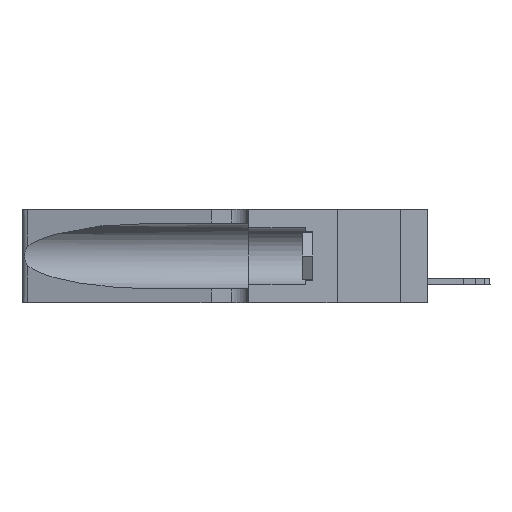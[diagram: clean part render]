
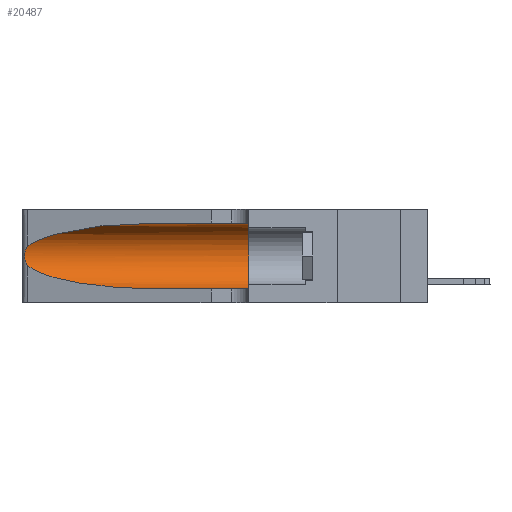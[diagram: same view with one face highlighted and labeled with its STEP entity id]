
A CAD part, left-side view. The second image highlights one B-rep face of the part: STEP entity #20487.
In plain terms, the highlighted cylindrical face has radius 3.308 mm (diameter 6.617 mm), a partial arc.
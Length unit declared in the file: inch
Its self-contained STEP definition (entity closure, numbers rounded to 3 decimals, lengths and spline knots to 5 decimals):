
#1 = CARTESIAN_POINT ( 'NONE',  ( 0.25555, 1.22994, 0.2215 ) ) ;
#87 = CARTESIAN_POINT ( 'NONE',  ( 0.1305, 0.35, 0.185 ) ) ;
#368 = B_SPLINE_CURVE_WITH_KNOTS ( 'NONE', 3,
 ( #2170, #1, #12106, #12592, #8756, #17978, #19268, #5569, #2104, #13566, #16265, #23050, #21181, #4207 ),
 .UNSPECIFIED., .F., .F.,
 ( 4, 2, 2, 2, 2, 2, 4 ),
 ( 0., 0.00027, 0.00053, 0.00107, 0.0016, 0.00187, 0.00214 ),
 .UNSPECIFIED. ) ;
#1150 = AXIS2_PLACEMENT_3D ( 'NONE', #9232, #19869, #3007 ) ;
#2104 = CARTESIAN_POINT ( 'NONE',  ( 0.26017, 1.23833, 0.17102 ) ) ;
#2170 = CARTESIAN_POINT ( 'NONE',  ( 0.25487, 1.22718, 0.22369 ) ) ;
#2233 = EDGE_CURVE ( 'NONE', #18518, #26636, #19519, .T. ) ;
#2275 = CARTESIAN_POINT ( 'NONE',  ( 0.18966, 0.96281, 0.31525 ) ) ;
#2387 = CARTESIAN_POINT ( 'NONE',  ( 0.18966, 0.96281, 0.05475 ) ) ;
#2442 = CARTESIAN_POINT ( 'NONE',  ( 0.25487, 1.22718, 0.14631 ) ) ;
#2450 = CARTESIAN_POINT ( 'NONE',  ( 0.25487, 1.22718, 0.22369 ) ) ;
#2698 = EDGE_CURVE ( 'NONE', #15589, #18518, #368, .T. ) ;
#3007 = DIRECTION ( 'NONE',  ( 0., 0., -1. ) ) ;
#3049 = CARTESIAN_POINT ( 'NONE',  ( 0.1305, 0.72297, 0.05475 ) ) ;
#4207 = CARTESIAN_POINT ( 'NONE',  ( 0.25487, 1.22718, 0.14631 ) ) ;
#4606 = ORIENTED_EDGE ( 'NONE', *, *, #25738, .F. ) ;
#5569 = CARTESIAN_POINT ( 'NONE',  ( 0.26075, 1.23896, 0.178 ) ) ;
#6267 = VERTEX_POINT ( 'NONE', #27074 ) ;
#6815 = VERTEX_POINT ( 'NONE', #14926 ) ;
#8517 = VECTOR ( 'NONE', #13620, 39.37008 ) ;
#8756 = CARTESIAN_POINT ( 'NONE',  ( 0.25854, 1.2359, 0.20912 ) ) ;
#9232 = CARTESIAN_POINT ( 'NONE',  ( 0.1305, 1.61858, 0.185 ) ) ;
#9313 = CARTESIAN_POINT ( 'NONE',  ( 0.1305, 1.61858, 0.05475 ) ) ;
#9803 = FACE_OUTER_BOUND ( 'NONE', #13865, .T. ) ;
#9966 = ORIENTED_EDGE ( 'NONE', *, *, #25538, .F. ) ;
#10868 = CARTESIAN_POINT ( 'NONE',  ( 0.25487, 1.22718, 0.14631 ) ) ;
#11461 = ORIENTED_EDGE ( 'NONE', *, *, #26034, .T. ) ;
#11840 = CIRCLE ( 'NONE', #14511, 0.13025 ) ;
#12106 = CARTESIAN_POINT ( 'NONE',  ( 0.25639, 1.23184, 0.21858 ) ) ;
#12592 = CARTESIAN_POINT ( 'NONE',  ( 0.25787, 1.23484, 0.2124 ) ) ;
#13566 = CARTESIAN_POINT ( 'NONE',  ( 0.25856, 1.23593, 0.16098 ) ) ;
#13620 = DIRECTION ( 'NONE',  ( 0., -1., 0. ) ) ;
#13839 = LINE ( 'NONE', #9313, #8517 ) ;
#13865 = EDGE_LOOP ( 'NONE', ( #27558, #18301, #23616, #11461, #4606, #9966 ) ) ;
#14511 = AXIS2_PLACEMENT_3D ( 'NONE', #87, #16988, #17082 ) ;
#14576 = LINE ( 'NONE', #24652, #18218 ) ;
#14824 = CYLINDRICAL_SURFACE ( 'NONE', #1150, 0.13025 ) ;
#14926 = CARTESIAN_POINT ( 'NONE',  ( 0.1305, 0.35, 0.31525 ) ) ;
#15065 = CARTESIAN_POINT ( 'NONE',  ( 0.1305, 0.72297, 0.31525 ) ) ;
#15589 = VERTEX_POINT ( 'NONE', #22653 ) ;
#16265 = CARTESIAN_POINT ( 'NONE',  ( 0.25789, 1.23486, 0.15765 ) ) ;
#16988 = DIRECTION ( 'NONE',  ( 0., 1., 0. ) ) ;
#17082 = DIRECTION ( 'NONE',  ( 0., 0., 1. ) ) ;
#17089 = CARTESIAN_POINT ( 'NONE',  ( 0.2373, 1.15595, 0.28018 ) ) ;
#17588 = CARTESIAN_POINT ( 'NONE',  ( 0.2373, 1.15595, 0.08982 ) ) ;
#17816 =( BOUNDED_CURVE ( )  B_SPLINE_CURVE ( 3, ( #15065, #2275, #17089, #2450 ),
 .UNSPECIFIED., .F., .F. ) 
 B_SPLINE_CURVE_WITH_KNOTS ( ( 4, 4 ),
 ( 1.5708, 2.84003 ),
 .UNSPECIFIED. ) 
 CURVE ( )  GEOMETRIC_REPRESENTATION_ITEM ( )  RATIONAL_B_SPLINE_CURVE ( ( 1., 0.87, 0.87, 1. ) ) 
 REPRESENTATION_ITEM ( '' )  );
#17978 = CARTESIAN_POINT ( 'NONE',  ( 0.26018, 1.23835, 0.19895 ) ) ;
#18218 = VECTOR ( 'NONE', #27413, 39.37008 ) ;
#18301 = ORIENTED_EDGE ( 'NONE', *, *, #2698, .T. ) ;
#18518 = VERTEX_POINT ( 'NONE', #2442 ) ;
#18757 = VERTEX_POINT ( 'NONE', #24623 ) ;
#19268 = CARTESIAN_POINT ( 'NONE',  ( 0.26075, 1.23896, 0.19203 ) ) ;
#19519 =( BOUNDED_CURVE ( )  B_SPLINE_CURVE ( 3, ( #10868, #17588, #2387, #21607 ),
 .UNSPECIFIED., .F., .T. ) 
 B_SPLINE_CURVE_WITH_KNOTS ( ( 4, 4 ),
 ( 3.44316, 4.71239 ),
 .UNSPECIFIED. ) 
 CURVE ( )  GEOMETRIC_REPRESENTATION_ITEM ( )  RATIONAL_B_SPLINE_CURVE ( ( 1., 0.87, 0.87, 1. ) ) 
 REPRESENTATION_ITEM ( '' )  );
#19869 = DIRECTION ( 'NONE',  ( 0., -1., 0. ) ) ;
#20487 = ADVANCED_FACE ( 'NONE', ( #9803 ), #14824, .F. ) ;
#21116 = EDGE_CURVE ( 'NONE', #18757, #15589, #17816, .T. ) ;
#21181 = CARTESIAN_POINT ( 'NONE',  ( 0.25555, 1.22993, 0.14849 ) ) ;
#21607 = CARTESIAN_POINT ( 'NONE',  ( 0.1305, 0.72297, 0.05475 ) ) ;
#22653 = CARTESIAN_POINT ( 'NONE',  ( 0.25487, 1.22718, 0.22369 ) ) ;
#23050 = CARTESIAN_POINT ( 'NONE',  ( 0.25639, 1.23186, 0.15144 ) ) ;
#23616 = ORIENTED_EDGE ( 'NONE', *, *, #2233, .T. ) ;
#24623 = CARTESIAN_POINT ( 'NONE',  ( 0.1305, 0.72297, 0.31525 ) ) ;
#24652 = CARTESIAN_POINT ( 'NONE',  ( 0.1305, 1.61858, 0.31525 ) ) ;
#25538 = EDGE_CURVE ( 'NONE', #18757, #6815, #14576, .T. ) ;
#25738 = EDGE_CURVE ( 'NONE', #6815, #6267, #11840, .T. ) ;
#26034 = EDGE_CURVE ( 'NONE', #26636, #6267, #13839, .T. ) ;
#26636 = VERTEX_POINT ( 'NONE', #3049 ) ;
#27074 = CARTESIAN_POINT ( 'NONE',  ( 0.1305, 0.35, 0.05475 ) ) ;
#27413 = DIRECTION ( 'NONE',  ( 0., -1., 0. ) ) ;
#27558 = ORIENTED_EDGE ( 'NONE', *, *, #21116, .T. ) ;
